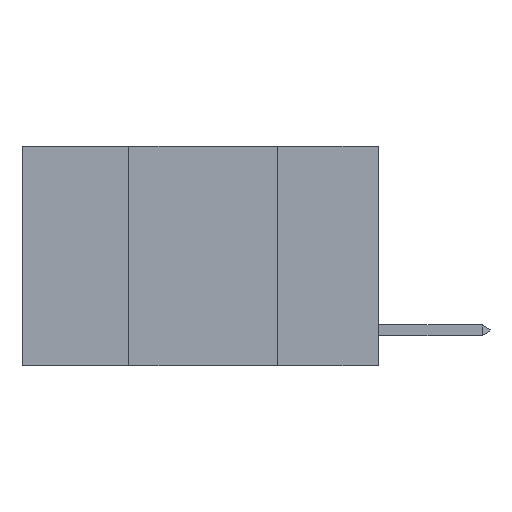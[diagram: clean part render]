
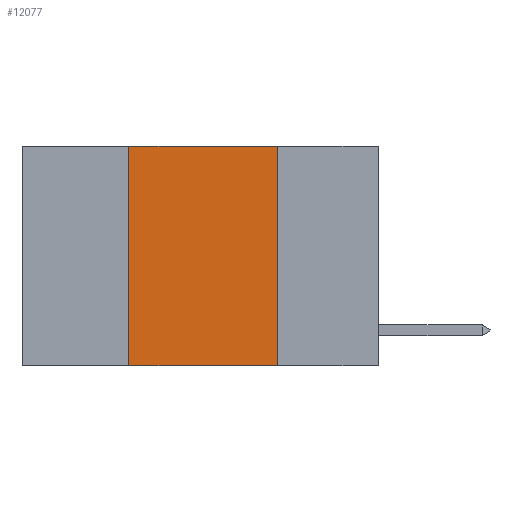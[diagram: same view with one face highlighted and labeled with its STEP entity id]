
A CAD part, left-side view. The second image highlights one B-rep face of the part: STEP entity #12077.
In plain terms, the highlighted planar face has unit normal (-1, 0, 0).
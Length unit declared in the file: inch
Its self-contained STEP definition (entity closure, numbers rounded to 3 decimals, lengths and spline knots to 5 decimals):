
#515 = DIRECTION ( 'NONE',  ( 0., 0., -1. ) ) ;
#1397 = LINE ( 'NONE', #17179, #6236 ) ;
#1986 = EDGE_CURVE ( 'NONE', #8796, #17575, #12961, .T. ) ;
#4106 = PLANE ( 'NONE',  #5762 ) ;
#4680 = CARTESIAN_POINT ( 'NONE',  ( 0., 0.17, 0. ) ) ;
#5762 = AXIS2_PLACEMENT_3D ( 'NONE', #8167, #21760, #10181 ) ;
#5791 = VECTOR ( 'NONE', #24587, 39.37008 ) ;
#6206 = VERTEX_POINT ( 'NONE', #18750 ) ;
#6236 = VECTOR ( 'NONE', #7400, 39.37008 ) ;
#7400 = DIRECTION ( 'NONE',  ( 0., -1., 0. ) ) ;
#7814 = EDGE_CURVE ( 'NONE', #7851, #6206, #9063, .T. ) ;
#7851 = VERTEX_POINT ( 'NONE', #4680 ) ;
#8167 = CARTESIAN_POINT ( 'NONE',  ( 0., 0.6, 0. ) ) ;
#8617 = EDGE_LOOP ( 'NONE', ( #16868, #21389, #24681, #12704 ) ) ;
#8796 = VERTEX_POINT ( 'NONE', #17488 ) ;
#8831 = CARTESIAN_POINT ( 'NONE',  ( 0., 0.42, 0. ) ) ;
#9063 = LINE ( 'NONE', #16524, #23938 ) ;
#9335 = FACE_OUTER_BOUND ( 'NONE', #8617, .T. ) ;
#10181 = DIRECTION ( 'NONE',  ( 0., 0., -1. ) ) ;
#11086 = CARTESIAN_POINT ( 'NONE',  ( 0., 0.6, 0. ) ) ;
#12077 = ADVANCED_FACE ( 'NONE', ( #9335 ), #4106, .F. ) ;
#12704 = ORIENTED_EDGE ( 'NONE', *, *, #24613, .T. ) ;
#12961 = LINE ( 'NONE', #8831, #17462 ) ;
#14198 = CARTESIAN_POINT ( 'NONE',  ( 0., 0.42, 0. ) ) ;
#14409 = EDGE_CURVE ( 'NONE', #17575, #7851, #17495, .T. ) ;
#14809 = DIRECTION ( 'NONE',  ( 0., 0., 1. ) ) ;
#16524 = CARTESIAN_POINT ( 'NONE',  ( 0., 0.17, 0. ) ) ;
#16868 = ORIENTED_EDGE ( 'NONE', *, *, #7814, .F. ) ;
#17179 = CARTESIAN_POINT ( 'NONE',  ( 0., 0.6, -0.37 ) ) ;
#17462 = VECTOR ( 'NONE', #14809, 39.37008 ) ;
#17488 = CARTESIAN_POINT ( 'NONE',  ( 0., 0.42, -0.37 ) ) ;
#17495 = LINE ( 'NONE', #11086, #5791 ) ;
#17575 = VERTEX_POINT ( 'NONE', #14198 ) ;
#18750 = CARTESIAN_POINT ( 'NONE',  ( 0., 0.17, -0.37 ) ) ;
#21389 = ORIENTED_EDGE ( 'NONE', *, *, #14409, .F. ) ;
#21760 = DIRECTION ( 'NONE',  ( 1., 0., 0. ) ) ;
#23938 = VECTOR ( 'NONE', #515, 39.37008 ) ;
#24587 = DIRECTION ( 'NONE',  ( 0., -1., 0. ) ) ;
#24613 = EDGE_CURVE ( 'NONE', #8796, #6206, #1397, .T. ) ;
#24681 = ORIENTED_EDGE ( 'NONE', *, *, #1986, .F. ) ;
